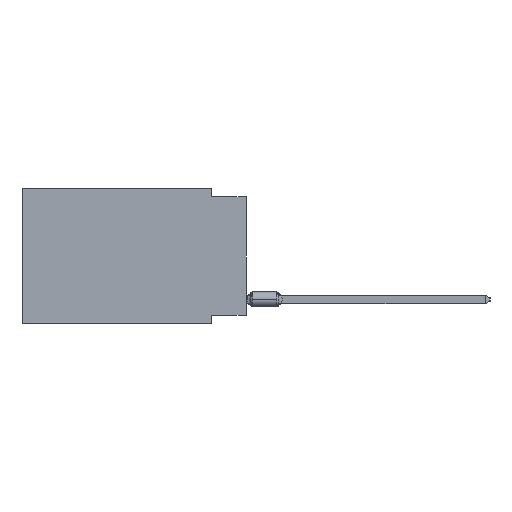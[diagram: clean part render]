
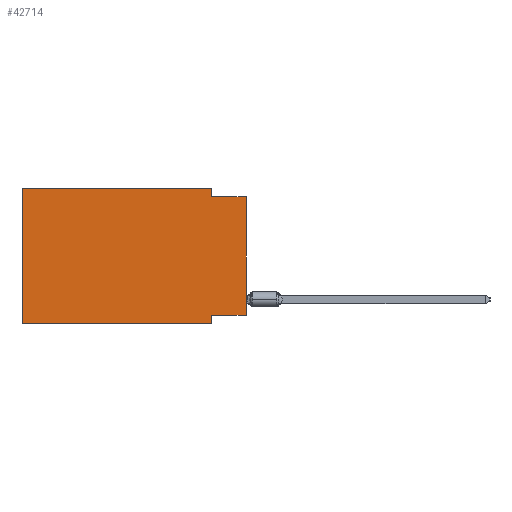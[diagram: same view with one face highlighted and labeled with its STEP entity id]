
A CAD part, left-side view. The second image highlights one B-rep face of the part: STEP entity #42714.
In plain terms, the highlighted planar face has unit normal (-1, 0, 0).
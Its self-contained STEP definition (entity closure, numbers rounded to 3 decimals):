
#17 = FACE_OUTER_BOUND ( 'NONE', #33746, .T. ) ;
#649 = DIRECTION ( 'NONE',  ( 0., 1., 0. ) ) ;
#2145 = ORIENTED_EDGE ( 'NONE', *, *, #36782, .F. ) ;
#2322 = ORIENTED_EDGE ( 'NONE', *, *, #3612, .F. ) ;
#3612 = EDGE_CURVE ( 'NONE', #14581, #20403, #29691, .T. ) ;
#3653 = LINE ( 'NONE', #10803, #42736 ) ;
#4474 = DIRECTION ( 'NONE',  ( 0., -1., 0. ) ) ;
#4558 = CARTESIAN_POINT ( 'NONE',  ( 0., 0., -0.635 ) ) ;
#5843 = ORIENTED_EDGE ( 'NONE', *, *, #27471, .F. ) ;
#6032 = CARTESIAN_POINT ( 'NONE',  ( 0., 16.383, -9.906 ) ) ;
#6648 = LINE ( 'NONE', #32555, #27015 ) ;
#6677 = CARTESIAN_POINT ( 'NONE',  ( 0., 0., -0.635 ) ) ;
#7017 = ORIENTED_EDGE ( 'NONE', *, *, #24178, .F. ) ;
#7200 = ORIENTED_EDGE ( 'NONE', *, *, #26040, .F. ) ;
#7308 = CARTESIAN_POINT ( 'NONE',  ( 0., 2.54, -9.906 ) ) ;
#10803 = CARTESIAN_POINT ( 'NONE',  ( 0., 2.54, 0. ) ) ;
#13636 = ORIENTED_EDGE ( 'NONE', *, *, #41605, .T. ) ;
#13696 = ORIENTED_EDGE ( 'NONE', *, *, #31818, .F. ) ;
#14581 = VERTEX_POINT ( 'NONE', #45066 ) ;
#15485 = VERTEX_POINT ( 'NONE', #6032 ) ;
#16033 = VERTEX_POINT ( 'NONE', #6677 ) ;
#16394 = CARTESIAN_POINT ( 'NONE',  ( 0., 2.54, -0.635 ) ) ;
#16447 = CARTESIAN_POINT ( 'NONE',  ( 0., 16.383, 0. ) ) ;
#17013 = VECTOR ( 'NONE', #22678, 1000. ) ;
#17099 = CARTESIAN_POINT ( 'NONE',  ( 0., 2.54, 0. ) ) ;
#17759 = CARTESIAN_POINT ( 'NONE',  ( 0., 2.54, -9.271 ) ) ;
#18049 = DIRECTION ( 'NONE',  ( 0., 0., 1. ) ) ;
#18293 = CARTESIAN_POINT ( 'NONE',  ( 0., 0., -9.271 ) ) ;
#20403 = VERTEX_POINT ( 'NONE', #17099 ) ;
#20665 = VERTEX_POINT ( 'NONE', #7308 ) ;
#20921 = VECTOR ( 'NONE', #44743, 1000. ) ;
#22101 = VERTEX_POINT ( 'NONE', #16394 ) ;
#22542 = CARTESIAN_POINT ( 'NONE',  ( 0., 16.383, 0. ) ) ;
#22643 = ORIENTED_EDGE ( 'NONE', *, *, #46852, .T. ) ;
#22678 = DIRECTION ( 'NONE',  ( 0., 0., 1. ) ) ;
#22973 = DIRECTION ( 'NONE',  ( 0., -1., 0. ) ) ;
#24178 = EDGE_CURVE ( 'NONE', #15485, #14581, #45675, .T. ) ;
#26040 = EDGE_CURVE ( 'NONE', #22101, #16033, #37145, .T. ) ;
#27015 = VECTOR ( 'NONE', #18049, 1000. ) ;
#27471 = EDGE_CURVE ( 'NONE', #20403, #22101, #3653, .T. ) ;
#28545 = VERTEX_POINT ( 'NONE', #18293 ) ;
#28667 = VECTOR ( 'NONE', #39966, 1000. ) ;
#29587 = DIRECTION ( 'NONE',  ( 0., 0., -1. ) ) ;
#29691 = LINE ( 'NONE', #22542, #40974 ) ;
#31818 = EDGE_CURVE ( 'NONE', #28545, #39210, #40392, .T. ) ;
#32555 = CARTESIAN_POINT ( 'NONE',  ( 0., 0., 0. ) ) ;
#32740 = VECTOR ( 'NONE', #649, 1000. ) ;
#33242 = CARTESIAN_POINT ( 'NONE',  ( 0., 0., -9.271 ) ) ;
#33568 = PLANE ( 'NONE',  #39487 ) ;
#33746 = EDGE_LOOP ( 'NONE', ( #13636, #7200, #5843, #2322, #7017, #22643, #2145, #13696 ) ) ;
#36414 = DIRECTION ( 'NONE',  ( 0., 0., -1. ) ) ;
#36782 = EDGE_CURVE ( 'NONE', #39210, #20665, #37108, .T. ) ;
#37108 = LINE ( 'NONE', #39744, #28667 ) ;
#37145 = LINE ( 'NONE', #4558, #20921 ) ;
#37504 = VECTOR ( 'NONE', #22973, 1000. ) ;
#39210 = VERTEX_POINT ( 'NONE', #17759 ) ;
#39487 = AXIS2_PLACEMENT_3D ( 'NONE', #40923, #43789, #36414 ) ;
#39744 = CARTESIAN_POINT ( 'NONE',  ( 0., 2.54, -9.906 ) ) ;
#39966 = DIRECTION ( 'NONE',  ( 0., 0., -1. ) ) ;
#40392 = LINE ( 'NONE', #33242, #32740 ) ;
#40923 = CARTESIAN_POINT ( 'NONE',  ( 0., 16.383, 0. ) ) ;
#40974 = VECTOR ( 'NONE', #4474, 1000. ) ;
#41058 = CARTESIAN_POINT ( 'NONE',  ( 0., 16.383, -9.906 ) ) ;
#41297 = LINE ( 'NONE', #41058, #37504 ) ;
#41605 = EDGE_CURVE ( 'NONE', #28545, #16033, #6648, .T. ) ;
#42714 = ADVANCED_FACE ( 'NONE', ( #17 ), #33568, .F. ) ;
#42736 = VECTOR ( 'NONE', #29587, 1000. ) ;
#43789 = DIRECTION ( 'NONE',  ( 1., 0., 0. ) ) ;
#44743 = DIRECTION ( 'NONE',  ( 0., -1., 0. ) ) ;
#45066 = CARTESIAN_POINT ( 'NONE',  ( 0., 16.383, 0. ) ) ;
#45675 = LINE ( 'NONE', #16447, #17013 ) ;
#46852 = EDGE_CURVE ( 'NONE', #15485, #20665, #41297, .T. ) ;
